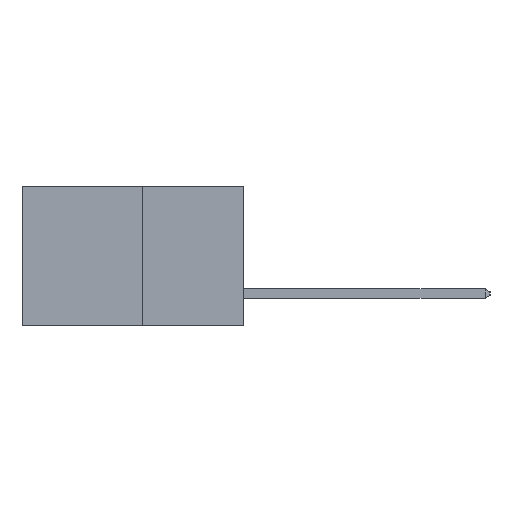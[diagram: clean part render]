
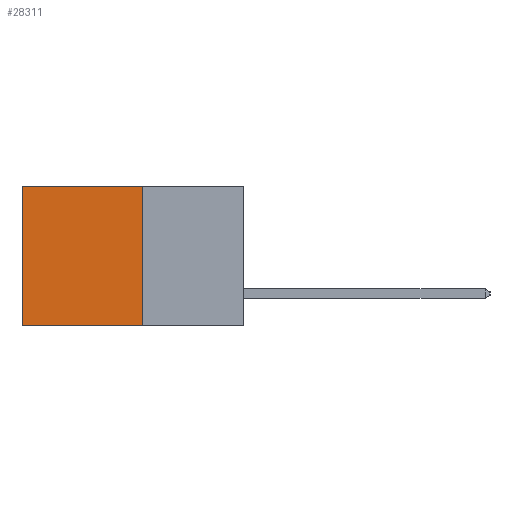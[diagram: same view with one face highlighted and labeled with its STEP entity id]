
A CAD part, left-side view. The second image highlights one B-rep face of the part: STEP entity #28311.
In plain terms, the highlighted planar face has unit normal (-1, 0, 0).
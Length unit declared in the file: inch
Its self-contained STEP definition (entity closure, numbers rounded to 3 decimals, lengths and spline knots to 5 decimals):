
#778 = CARTESIAN_POINT ( 'NONE',  ( 0.277, 0.59, 0. ) ) ;
#2693 = EDGE_CURVE ( 'NONE', #18429, #3700, #14430, .T. ) ;
#3142 = EDGE_CURVE ( 'NONE', #29236, #3700, #20585, .T. ) ;
#3700 = VERTEX_POINT ( 'NONE', #9441 ) ;
#5402 = EDGE_CURVE ( 'NONE', #21969, #18429, #19454, .T. ) ;
#8112 = CARTESIAN_POINT ( 'NONE',  ( 0.277, 0.27, 0. ) ) ;
#8329 = VECTOR ( 'NONE', #22344, 39.37008 ) ;
#8818 = CARTESIAN_POINT ( 'NONE',  ( 0.277, 0.27, -0.37 ) ) ;
#9441 = CARTESIAN_POINT ( 'NONE',  ( 0.277, 0.59, -0.37 ) ) ;
#11140 = PLANE ( 'NONE',  #16402 ) ;
#11254 = ORIENTED_EDGE ( 'NONE', *, *, #3142, .T. ) ;
#11542 = ORIENTED_EDGE ( 'NONE', *, *, #12339, .T. ) ;
#12339 = EDGE_CURVE ( 'NONE', #21969, #29236, #24663, .T. ) ;
#12773 = CARTESIAN_POINT ( 'NONE',  ( 0.277, 0.27, -0.37 ) ) ;
#13308 = VECTOR ( 'NONE', #29785, 39.37008 ) ;
#13435 = DIRECTION ( 'NONE',  ( 0., 0., -1. ) ) ;
#13596 = CARTESIAN_POINT ( 'NONE',  ( 0.277, 0.59, -0.37 ) ) ;
#13908 = CARTESIAN_POINT ( 'NONE',  ( 0.277, 0.27, -0.37 ) ) ;
#14407 = VECTOR ( 'NONE', #24066, 39.37008 ) ;
#14430 = LINE ( 'NONE', #12773, #8329 ) ;
#15030 = DIRECTION ( 'NONE',  ( 0., 1., 0. ) ) ;
#16402 = AXIS2_PLACEMENT_3D ( 'NONE', #8818, #17984, #13435 ) ;
#17667 = ORIENTED_EDGE ( 'NONE', *, *, #5402, .F. ) ;
#17984 = DIRECTION ( 'NONE',  ( 1., 0., 0. ) ) ;
#18429 = VERTEX_POINT ( 'NONE', #13908 ) ;
#18551 = VECTOR ( 'NONE', #15030, 39.37008 ) ;
#18924 = FACE_OUTER_BOUND ( 'NONE', #19219, .T. ) ;
#19219 = EDGE_LOOP ( 'NONE', ( #11254, #25704, #17667, #11542 ) ) ;
#19454 = LINE ( 'NONE', #29121, #13308 ) ;
#20585 = LINE ( 'NONE', #13596, #14407 ) ;
#21969 = VERTEX_POINT ( 'NONE', #22462 ) ;
#22344 = DIRECTION ( 'NONE',  ( 0., 1., 0. ) ) ;
#22462 = CARTESIAN_POINT ( 'NONE',  ( 0.277, 0.27, 0. ) ) ;
#24066 = DIRECTION ( 'NONE',  ( 0., 0., -1. ) ) ;
#24663 = LINE ( 'NONE', #8112, #18551 ) ;
#25704 = ORIENTED_EDGE ( 'NONE', *, *, #2693, .F. ) ;
#28311 = ADVANCED_FACE ( 'NONE', ( #18924 ), #11140, .F. ) ;
#29121 = CARTESIAN_POINT ( 'NONE',  ( 0.277, 0.27, -0.37 ) ) ;
#29236 = VERTEX_POINT ( 'NONE', #778 ) ;
#29785 = DIRECTION ( 'NONE',  ( 0., 0., -1. ) ) ;
